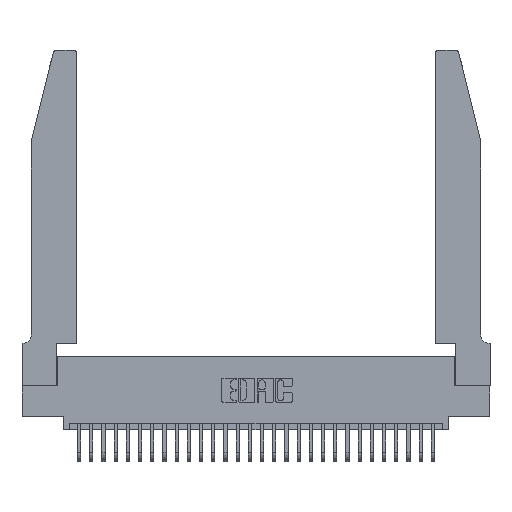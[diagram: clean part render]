
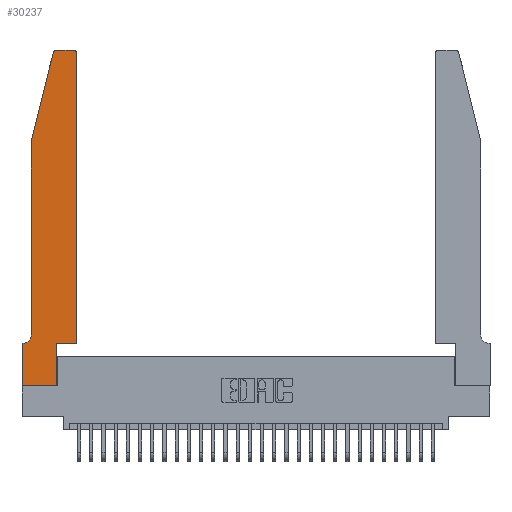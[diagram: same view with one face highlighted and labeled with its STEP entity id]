
A CAD part, top view. The second image highlights one B-rep face of the part: STEP entity #30237.
In plain terms, the highlighted planar face has unit normal (0, 0, 1).
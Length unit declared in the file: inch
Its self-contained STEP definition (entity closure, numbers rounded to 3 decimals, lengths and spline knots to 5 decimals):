
#412 = EDGE_CURVE ( 'NONE', #21977, #16653, #23628, .T. ) ;
#427 = ORIENTED_EDGE ( 'NONE', *, *, #20556, .T. ) ;
#513 = AXIS2_PLACEMENT_3D ( 'NONE', #17208, #2482, #19630 ) ;
#997 = CARTESIAN_POINT ( 'NONE',  ( 0.0755, 0.42, 0.37 ) ) ;
#1493 = CARTESIAN_POINT ( 'NONE',  ( 0.0755, 2., 0.37 ) ) ;
#1563 = DIRECTION ( 'NONE',  ( -1., 0., 0. ) ) ;
#1969 = CARTESIAN_POINT ( 'NONE',  ( 0.4505, 0.35, 0.37 ) ) ;
#2250 = DIRECTION ( 'NONE',  ( -1., 0., 0. ) ) ;
#2253 = CARTESIAN_POINT ( 'NONE',  ( 0.2865, 0.35, 0.37 ) ) ;
#2482 = DIRECTION ( 'NONE',  ( 0., 0., 1. ) ) ;
#3384 = CARTESIAN_POINT ( 'NONE',  ( 0.2865, 0., 0.37 ) ) ;
#3556 = ORIENTED_EDGE ( 'NONE', *, *, #412, .T. ) ;
#3985 = DIRECTION ( 'NONE',  ( 1., 0., 0. ) ) ;
#4021 = DIRECTION ( 'NONE',  ( 0., 0., -1. ) ) ;
#4244 = PLANE ( 'NONE',  #22265 ) ;
#4746 = DIRECTION ( 'NONE',  ( 0., 0., 1. ) ) ;
#4768 = VERTEX_POINT ( 'NONE', #1493 ) ;
#4784 = VECTOR ( 'NONE', #25546, 39.37008 ) ;
#4839 = CARTESIAN_POINT ( 'NONE',  ( 0.284, 2.75, 0.37 ) ) ;
#5017 = LINE ( 'NONE', #12132, #10795 ) ;
#5346 = VECTOR ( 'NONE', #21851, 39.37008 ) ;
#5731 = EDGE_LOOP ( 'NONE', ( #20284, #30101, #31600, #6612, #15121, #31316, #7856, #3556, #29148, #427, #14139, #30950 ) ) ;
#6612 = ORIENTED_EDGE ( 'NONE', *, *, #8029, .T. ) ;
#7139 = LINE ( 'NONE', #19319, #12904 ) ;
#7789 = EDGE_CURVE ( 'NONE', #17201, #21977, #11340, .T. ) ;
#7850 = VERTEX_POINT ( 'NONE', #18473 ) ;
#7856 = ORIENTED_EDGE ( 'NONE', *, *, #7789, .T. ) ;
#8029 = EDGE_CURVE ( 'NONE', #4768, #12020, #30935, .T. ) ;
#9209 = DIRECTION ( 'NONE',  ( 0., 0., 1. ) ) ;
#9333 = VERTEX_POINT ( 'NONE', #17129 ) ;
#10074 = FACE_OUTER_BOUND ( 'NONE', #5731, .T. ) ;
#10473 = CARTESIAN_POINT ( 'NONE',  ( 0.4205, 2.75, 0.37 ) ) ;
#10491 = EDGE_CURVE ( 'NONE', #24248, #21124, #23616, .T. ) ;
#10678 = EDGE_CURVE ( 'NONE', #16653, #7850, #24742, .T. ) ;
#10725 = EDGE_CURVE ( 'NONE', #21124, #17730, #11105, .T. ) ;
#10752 = VECTOR ( 'NONE', #3985, 39.37008 ) ;
#10795 = VECTOR ( 'NONE', #2250, 39.37008 ) ;
#11096 = AXIS2_PLACEMENT_3D ( 'NONE', #18672, #4021, #21076 ) ;
#11105 = CIRCLE ( 'NONE', #513, 0.03 ) ;
#11340 = LINE ( 'NONE', #23151, #4784 ) ;
#12020 = VERTEX_POINT ( 'NONE', #997 ) ;
#12132 = CARTESIAN_POINT ( 'NONE',  ( 0.0755, 0.35, 0.37 ) ) ;
#12312 = EDGE_CURVE ( 'NONE', #17730, #4768, #7139, .T. ) ;
#12494 = EDGE_CURVE ( 'NONE', #16146, #27959, #21189, .T. ) ;
#12904 = VECTOR ( 'NONE', #28990, 39.37008 ) ;
#13541 = CARTESIAN_POINT ( 'NONE',  ( 0.4505, 0.35, 0.37 ) ) ;
#14139 = ORIENTED_EDGE ( 'NONE', *, *, #12494, .T. ) ;
#14800 = VECTOR ( 'NONE', #17534, 39.37008 ) ;
#15092 = CARTESIAN_POINT ( 'NONE',  ( 0., 0.35, 0.37 ) ) ;
#15121 = ORIENTED_EDGE ( 'NONE', *, *, #16818, .T. ) ;
#15124 = CARTESIAN_POINT ( 'NONE',  ( 0.4505, 0.35, 0.37 ) ) ;
#16146 = VERTEX_POINT ( 'NONE', #13541 ) ;
#16653 = VERTEX_POINT ( 'NONE', #3384 ) ;
#16818 = EDGE_CURVE ( 'NONE', #12020, #9333, #21142, .T. ) ;
#17129 = CARTESIAN_POINT ( 'NONE',  ( 0.0055, 0.35, 0.37 ) ) ;
#17201 = VERTEX_POINT ( 'NONE', #15092 ) ;
#17208 = CARTESIAN_POINT ( 'NONE',  ( 0.284, 2.72, 0.37 ) ) ;
#17534 = DIRECTION ( 'NONE',  ( 0., 1., 0. ) ) ;
#17730 = VERTEX_POINT ( 'NONE', #28922 ) ;
#18473 = CARTESIAN_POINT ( 'NONE',  ( 0.2865, 0.35, 0.37 ) ) ;
#18672 = CARTESIAN_POINT ( 'NONE',  ( 0.0055, 0.42, 0.37 ) ) ;
#19090 = CARTESIAN_POINT ( 'NONE',  ( 0.0755, 2., 0.37 ) ) ;
#19319 = CARTESIAN_POINT ( 'NONE',  ( 0.0755, 2., 0.37 ) ) ;
#19350 = CARTESIAN_POINT ( 'NONE',  ( 0.4205, 2.72, 0.37 ) ) ;
#19630 = DIRECTION ( 'NONE',  ( 1., 0., 0. ) ) ;
#19949 = EDGE_CURVE ( 'NONE', #9333, #17201, #5017, .T. ) ;
#20284 = ORIENTED_EDGE ( 'NONE', *, *, #10491, .T. ) ;
#20556 = EDGE_CURVE ( 'NONE', #7850, #16146, #22912, .T. ) ;
#21076 = DIRECTION ( 'NONE',  ( -1., 0., 0. ) ) ;
#21124 = VERTEX_POINT ( 'NONE', #4839 ) ;
#21142 = CIRCLE ( 'NONE', #11096, 0.07 ) ;
#21189 = LINE ( 'NONE', #15124, #14800 ) ;
#21207 = CARTESIAN_POINT ( 'NONE',  ( 0.2605, 2.75, 0.37 ) ) ;
#21702 = DIRECTION ( 'NONE',  ( 1., 0., 0. ) ) ;
#21775 = DIRECTION ( 'NONE',  ( 1., 0., 0. ) ) ;
#21851 = DIRECTION ( 'NONE',  ( 0., 1., 0. ) ) ;
#21977 = VERTEX_POINT ( 'NONE', #25111 ) ;
#22265 = AXIS2_PLACEMENT_3D ( 'NONE', #23742, #9209, #26158 ) ;
#22912 = LINE ( 'NONE', #1969, #27757 ) ;
#23151 = CARTESIAN_POINT ( 'NONE',  ( 0., 0., 0.37 ) ) ;
#23378 = CIRCLE ( 'NONE', #28062, 0.03 ) ;
#23616 = LINE ( 'NONE', #21207, #29227 ) ;
#23628 = LINE ( 'NONE', #31367, #10752 ) ;
#23742 = CARTESIAN_POINT ( 'NONE',  ( 0., 0.35, 0.37 ) ) ;
#23805 = VECTOR ( 'NONE', #23952, 39.37008 ) ;
#23952 = DIRECTION ( 'NONE',  ( 0., -1., 0. ) ) ;
#24248 = VERTEX_POINT ( 'NONE', #10473 ) ;
#24742 = LINE ( 'NONE', #2253, #5346 ) ;
#25111 = CARTESIAN_POINT ( 'NONE',  ( 0., 0., 0.37 ) ) ;
#25546 = DIRECTION ( 'NONE',  ( 0., -1., 0. ) ) ;
#26158 = DIRECTION ( 'NONE',  ( 1., 0., 0. ) ) ;
#26507 = EDGE_CURVE ( 'NONE', #27959, #24248, #23378, .T. ) ;
#27757 = VECTOR ( 'NONE', #21702, 39.37008 ) ;
#27959 = VERTEX_POINT ( 'NONE', #28183 ) ;
#28062 = AXIS2_PLACEMENT_3D ( 'NONE', #19350, #4746, #21775 ) ;
#28183 = CARTESIAN_POINT ( 'NONE',  ( 0.4505, 2.72, 0.37 ) ) ;
#28922 = CARTESIAN_POINT ( 'NONE',  ( 0.25487, 2.72718, 0.37 ) ) ;
#28990 = DIRECTION ( 'NONE',  ( -0.239, -0.971, 0. ) ) ;
#29148 = ORIENTED_EDGE ( 'NONE', *, *, #10678, .T. ) ;
#29227 = VECTOR ( 'NONE', #1563, 39.37008 ) ;
#30101 = ORIENTED_EDGE ( 'NONE', *, *, #10725, .T. ) ;
#30237 = ADVANCED_FACE ( 'NONE', ( #10074 ), #4244, .T. ) ;
#30935 = LINE ( 'NONE', #19090, #23805 ) ;
#30950 = ORIENTED_EDGE ( 'NONE', *, *, #26507, .T. ) ;
#31316 = ORIENTED_EDGE ( 'NONE', *, *, #19949, .T. ) ;
#31367 = CARTESIAN_POINT ( 'NONE',  ( 0., 0., 0.37 ) ) ;
#31600 = ORIENTED_EDGE ( 'NONE', *, *, #12312, .T. ) ;
